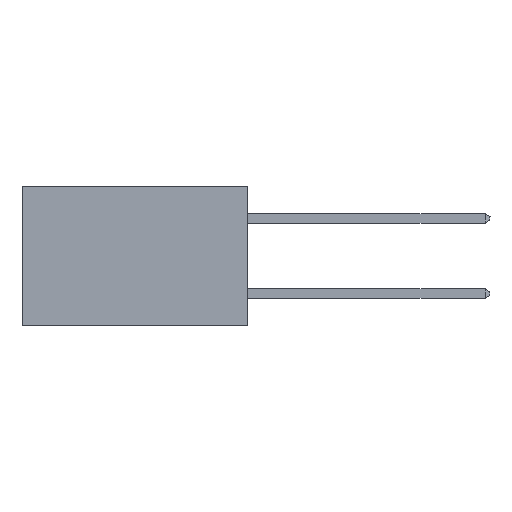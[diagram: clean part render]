
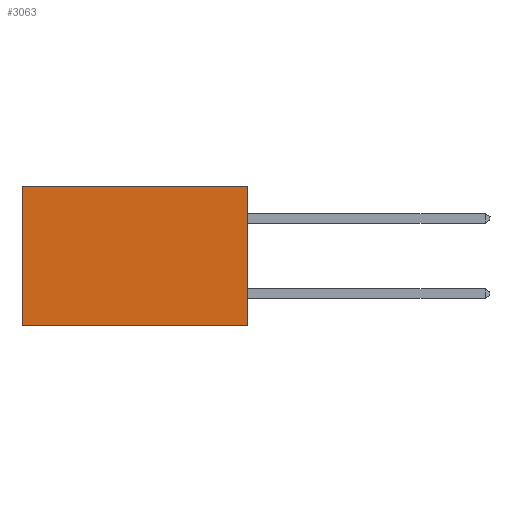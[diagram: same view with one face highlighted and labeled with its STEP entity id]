
A CAD part, left-side view. The second image highlights one B-rep face of the part: STEP entity #3063.
In plain terms, the highlighted planar face has unit normal (-1, 0, 0).
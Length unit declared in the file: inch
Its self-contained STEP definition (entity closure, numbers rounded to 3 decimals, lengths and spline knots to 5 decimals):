
#189 = ORIENTED_EDGE ( 'NONE', *, *, #4797, .F. ) ;
#290 = CARTESIAN_POINT ( 'NONE',  ( 0.298, 0., -0.37 ) ) ;
#645 = CARTESIAN_POINT ( 'NONE',  ( 0.298, 0., 0. ) ) ;
#971 = ORIENTED_EDGE ( 'NONE', *, *, #7915, .F. ) ;
#2053 = DIRECTION ( 'NONE',  ( 0., 0., -1. ) ) ;
#3063 = ADVANCED_FACE ( 'NONE', ( #7565 ), #8664, .F. ) ;
#3693 = DIRECTION ( 'NONE',  ( 0., 0., -1. ) ) ;
#4797 = EDGE_CURVE ( 'NONE', #12351, #7072, #8991, .T. ) ;
#4855 = DIRECTION ( 'NONE',  ( 0., 1., 0. ) ) ;
#5690 = CARTESIAN_POINT ( 'NONE',  ( 0.298, 0., 0. ) ) ;
#5965 = EDGE_CURVE ( 'NONE', #11206, #13145, #9883, .T. ) ;
#6332 = EDGE_CURVE ( 'NONE', #13145, #7072, #8560, .T. ) ;
#7072 = VERTEX_POINT ( 'NONE', #13649 ) ;
#7153 = CARTESIAN_POINT ( 'NONE',  ( 0.298, 0., 0. ) ) ;
#7286 = DIRECTION ( 'NONE',  ( 0., 1., 0. ) ) ;
#7457 = VECTOR ( 'NONE', #2053, 39.37008 ) ;
#7478 = CARTESIAN_POINT ( 'NONE',  ( 0.298, 0.6, 0. ) ) ;
#7565 = FACE_OUTER_BOUND ( 'NONE', #15215, .T. ) ;
#7915 = EDGE_CURVE ( 'NONE', #11206, #12351, #8291, .T. ) ;
#8068 = CARTESIAN_POINT ( 'NONE',  ( 0.298, 0.6, 0. ) ) ;
#8291 = LINE ( 'NONE', #645, #14814 ) ;
#8405 = CARTESIAN_POINT ( 'NONE',  ( 0.298, 0., 0. ) ) ;
#8560 = LINE ( 'NONE', #8068, #7457 ) ;
#8664 = PLANE ( 'NONE',  #12770 ) ;
#8991 = LINE ( 'NONE', #10969, #15326 ) ;
#9883 = LINE ( 'NONE', #7153, #15476 ) ;
#10969 = CARTESIAN_POINT ( 'NONE',  ( 0.298, 0., -0.37 ) ) ;
#11206 = VERTEX_POINT ( 'NONE', #5690 ) ;
#11989 = ORIENTED_EDGE ( 'NONE', *, *, #5965, .T. ) ;
#12066 = ORIENTED_EDGE ( 'NONE', *, *, #6332, .T. ) ;
#12351 = VERTEX_POINT ( 'NONE', #290 ) ;
#12770 = AXIS2_PLACEMENT_3D ( 'NONE', #8405, #13359, #3693 ) ;
#13145 = VERTEX_POINT ( 'NONE', #7478 ) ;
#13359 = DIRECTION ( 'NONE',  ( 1., 0., 0. ) ) ;
#13649 = CARTESIAN_POINT ( 'NONE',  ( 0.298, 0.6, -0.37 ) ) ;
#14814 = VECTOR ( 'NONE', #15001, 39.37008 ) ;
#15001 = DIRECTION ( 'NONE',  ( 0., 0., -1. ) ) ;
#15215 = EDGE_LOOP ( 'NONE', ( #12066, #189, #971, #11989 ) ) ;
#15326 = VECTOR ( 'NONE', #7286, 39.37008 ) ;
#15476 = VECTOR ( 'NONE', #4855, 39.37008 ) ;
